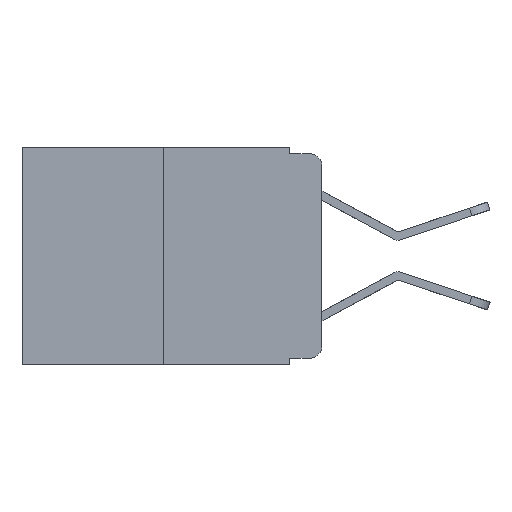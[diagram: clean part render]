
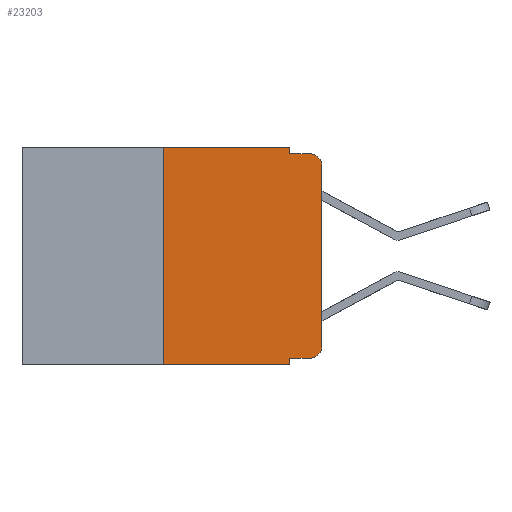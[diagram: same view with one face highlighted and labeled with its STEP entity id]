
A CAD part, left-side view. The second image highlights one B-rep face of the part: STEP entity #23203.
In plain terms, the highlighted planar face has unit normal (-1, 0, 0).
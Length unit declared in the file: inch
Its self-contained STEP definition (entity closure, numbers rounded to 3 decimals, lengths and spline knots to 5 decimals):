
#134 = LINE ( 'NONE', #5563, #4832 ) ;
#174 = VECTOR ( 'NONE', #14484, 39.37008 ) ;
#675 = ORIENTED_EDGE ( 'NONE', *, *, #12809, .T. ) ;
#903 = ORIENTED_EDGE ( 'NONE', *, *, #21468, .T. ) ;
#1195 = CARTESIAN_POINT ( 'NONE',  ( 0., 0.02, -0.313 ) ) ;
#1626 = CARTESIAN_POINT ( 'NONE',  ( 0., 0.25, 0. ) ) ;
#2197 = CARTESIAN_POINT ( 'NONE',  ( 0., 0.25, 0. ) ) ;
#2455 = CARTESIAN_POINT ( 'NONE',  ( 0., 0.051, -0.01 ) ) ;
#2551 = VERTEX_POINT ( 'NONE', #12127 ) ;
#2912 = AXIS2_PLACEMENT_3D ( 'NONE', #1195, #22596, #13876 ) ;
#3716 = CARTESIAN_POINT ( 'NONE',  ( 0., 0.473, 0. ) ) ;
#3819 = EDGE_CURVE ( 'NONE', #20706, #17470, #10705, .T. ) ;
#4175 = CARTESIAN_POINT ( 'NONE',  ( 0., 0.02, -0.333 ) ) ;
#4253 = DIRECTION ( 'NONE',  ( 0., 0., -1. ) ) ;
#4471 = ORIENTED_EDGE ( 'NONE', *, *, #20509, .F. ) ;
#4487 = CARTESIAN_POINT ( 'NONE',  ( 0., 0.051, -0.333 ) ) ;
#4556 = EDGE_CURVE ( 'NONE', #8166, #20706, #12962, .T. ) ;
#4832 = VECTOR ( 'NONE', #20119, 39.37008 ) ;
#5130 = CARTESIAN_POINT ( 'NONE',  ( 0., 0., 0. ) ) ;
#5294 = DIRECTION ( 'NONE',  ( 0., 0., 1. ) ) ;
#5312 = VERTEX_POINT ( 'NONE', #6516 ) ;
#5551 = CIRCLE ( 'NONE', #2912, 0.02 ) ;
#5563 = CARTESIAN_POINT ( 'NONE',  ( 0., 0.051, 0. ) ) ;
#5765 = AXIS2_PLACEMENT_3D ( 'NONE', #15170, #13395, #20643 ) ;
#6022 = DIRECTION ( 'NONE',  ( 0., 0., -1. ) ) ;
#6185 = CARTESIAN_POINT ( 'NONE',  ( 0., 0.25, -0.343 ) ) ;
#6516 = CARTESIAN_POINT ( 'NONE',  ( 0., 0.051, -0.343 ) ) ;
#7056 = ORIENTED_EDGE ( 'NONE', *, *, #3819, .F. ) ;
#7153 = EDGE_CURVE ( 'NONE', #21050, #2551, #13002, .T. ) ;
#7790 = CARTESIAN_POINT ( 'NONE',  ( 0., 0.051, 0. ) ) ;
#7834 = CARTESIAN_POINT ( 'NONE',  ( 0., 0.02, -0.01 ) ) ;
#8166 = VERTEX_POINT ( 'NONE', #6185 ) ;
#8247 = VECTOR ( 'NONE', #9933, 39.37008 ) ;
#8271 = VERTEX_POINT ( 'NONE', #4175 ) ;
#8284 = VERTEX_POINT ( 'NONE', #7834 ) ;
#8339 = CARTESIAN_POINT ( 'NONE',  ( 0., 0., -0.313 ) ) ;
#8360 = VERTEX_POINT ( 'NONE', #10477 ) ;
#9933 = DIRECTION ( 'NONE',  ( 0., -1., 0. ) ) ;
#9981 = VECTOR ( 'NONE', #6022, 39.37008 ) ;
#10039 = EDGE_CURVE ( 'NONE', #8271, #21050, #5551, .T. ) ;
#10069 = EDGE_CURVE ( 'NONE', #8166, #5312, #12331, .T. ) ;
#10151 = LINE ( 'NONE', #2455, #18514 ) ;
#10224 = VERTEX_POINT ( 'NONE', #14217 ) ;
#10233 = EDGE_CURVE ( 'NONE', #17470, #10224, #134, .T. ) ;
#10477 = CARTESIAN_POINT ( 'NONE',  ( 0., 0.051, -0.333 ) ) ;
#10705 = LINE ( 'NONE', #3716, #174 ) ;
#11450 = DIRECTION ( 'NONE',  ( 0., -1., 0. ) ) ;
#12127 = CARTESIAN_POINT ( 'NONE',  ( 0., 0., -0.03 ) ) ;
#12215 = CIRCLE ( 'NONE', #5765, 0.02 ) ;
#12324 = ORIENTED_EDGE ( 'NONE', *, *, #4556, .F. ) ;
#12331 = LINE ( 'NONE', #20980, #18404 ) ;
#12809 = EDGE_CURVE ( 'NONE', #8360, #8271, #15138, .T. ) ;
#12962 = LINE ( 'NONE', #2197, #19465 ) ;
#13002 = LINE ( 'NONE', #5130, #19236 ) ;
#13199 = EDGE_LOOP ( 'NONE', ( #21981, #903, #20365, #18299, #7056, #12324, #20629, #4471, #675, #21659 ) ) ;
#13247 = FACE_OUTER_BOUND ( 'NONE', #13199, .T. ) ;
#13395 = DIRECTION ( 'NONE',  ( -1., 0., 0. ) ) ;
#13876 = DIRECTION ( 'NONE',  ( 0., 0., -1. ) ) ;
#14217 = CARTESIAN_POINT ( 'NONE',  ( 0., 0.051, -0.01 ) ) ;
#14484 = DIRECTION ( 'NONE',  ( 0., -1., 0. ) ) ;
#14569 = EDGE_CURVE ( 'NONE', #10224, #8284, #10151, .T. ) ;
#14935 = DIRECTION ( 'NONE',  ( 1., 0., 0. ) ) ;
#15138 = LINE ( 'NONE', #4487, #8247 ) ;
#15147 = CARTESIAN_POINT ( 'NONE',  ( 0., 0.473, 0. ) ) ;
#15170 = CARTESIAN_POINT ( 'NONE',  ( 0., 0.02, -0.03 ) ) ;
#15885 = DIRECTION ( 'NONE',  ( 0., -1., 0. ) ) ;
#17470 = VERTEX_POINT ( 'NONE', #21753 ) ;
#17564 = AXIS2_PLACEMENT_3D ( 'NONE', #15147, #14935, #4253 ) ;
#18299 = ORIENTED_EDGE ( 'NONE', *, *, #10233, .F. ) ;
#18404 = VECTOR ( 'NONE', #15885, 39.37008 ) ;
#18514 = VECTOR ( 'NONE', #11450, 39.37008 ) ;
#19236 = VECTOR ( 'NONE', #21990, 39.37008 ) ;
#19465 = VECTOR ( 'NONE', #5294, 39.37008 ) ;
#20119 = DIRECTION ( 'NONE',  ( 0., 0., -1. ) ) ;
#20365 = ORIENTED_EDGE ( 'NONE', *, *, #14569, .F. ) ;
#20503 = PLANE ( 'NONE',  #17564 ) ;
#20509 = EDGE_CURVE ( 'NONE', #8360, #5312, #21895, .T. ) ;
#20629 = ORIENTED_EDGE ( 'NONE', *, *, #10069, .T. ) ;
#20643 = DIRECTION ( 'NONE',  ( 0., 0., -1. ) ) ;
#20706 = VERTEX_POINT ( 'NONE', #1626 ) ;
#20980 = CARTESIAN_POINT ( 'NONE',  ( 0., 0.473, -0.343 ) ) ;
#21050 = VERTEX_POINT ( 'NONE', #8339 ) ;
#21468 = EDGE_CURVE ( 'NONE', #2551, #8284, #12215, .T. ) ;
#21659 = ORIENTED_EDGE ( 'NONE', *, *, #10039, .T. ) ;
#21753 = CARTESIAN_POINT ( 'NONE',  ( 0., 0.051, 0. ) ) ;
#21895 = LINE ( 'NONE', #7790, #9981 ) ;
#21981 = ORIENTED_EDGE ( 'NONE', *, *, #7153, .T. ) ;
#21990 = DIRECTION ( 'NONE',  ( 0., 0., 1. ) ) ;
#22596 = DIRECTION ( 'NONE',  ( -1., 0., 0. ) ) ;
#23203 = ADVANCED_FACE ( 'NONE', ( #13247 ), #20503, .F. ) ;
